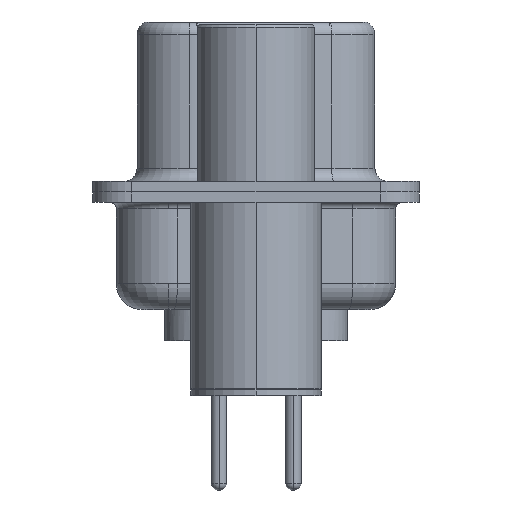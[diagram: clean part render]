
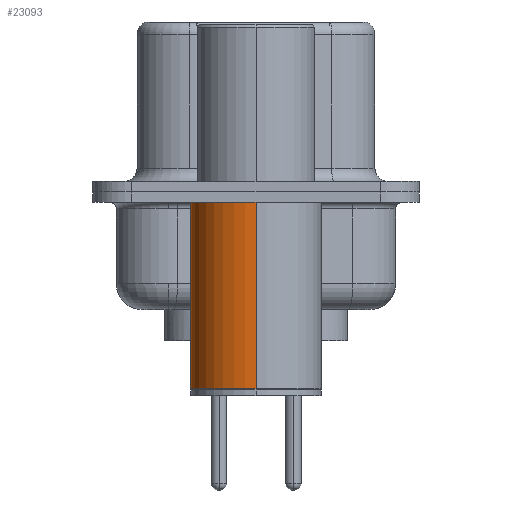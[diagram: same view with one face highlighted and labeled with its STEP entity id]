
A CAD part, left-side view. The second image highlights one B-rep face of the part: STEP entity #23093.
In plain terms, the highlighted cylindrical face has radius 2.5 mm (diameter 5 mm), a partial arc.
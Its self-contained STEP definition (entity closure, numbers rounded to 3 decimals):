
#487 = EDGE_CURVE ( 'NONE', #24582, #23290, #26613, .T. ) ;
#825 = CARTESIAN_POINT ( 'NONE',  ( 2.5, 0., -7.525 ) ) ;
#1726 = AXIS2_PLACEMENT_3D ( 'NONE', #17259, #23278, #4739 ) ;
#1856 = LINE ( 'NONE', #22162, #21550 ) ;
#3023 = CIRCLE ( 'NONE', #1726, 2.5 ) ;
#3059 = FACE_OUTER_BOUND ( 'NONE', #3855, .T. ) ;
#3647 = VERTEX_POINT ( 'NONE', #21560 ) ;
#3855 = EDGE_LOOP ( 'NONE', ( #4456, #26342, #9436, #11834 ) ) ;
#4138 = CARTESIAN_POINT ( 'NONE',  ( -2.5, 0., -0.4 ) ) ;
#4248 = VECTOR ( 'NONE', #20908, 1000. ) ;
#4456 = ORIENTED_EDGE ( 'NONE', *, *, #12412, .T. ) ;
#4544 = LINE ( 'NONE', #25258, #4248 ) ;
#4739 = DIRECTION ( 'NONE',  ( 1., 0., 0. ) ) ;
#4787 = EDGE_CURVE ( 'NONE', #20420, #24582, #4544, .T. ) ;
#4837 = CYLINDRICAL_SURFACE ( 'NONE', #8531, 2.5 ) ;
#8531 = AXIS2_PLACEMENT_3D ( 'NONE', #15748, #23914, #19706 ) ;
#9399 = CARTESIAN_POINT ( 'NONE',  ( 0., 0., -0.4 ) ) ;
#9436 = ORIENTED_EDGE ( 'NONE', *, *, #487, .F. ) ;
#11834 = ORIENTED_EDGE ( 'NONE', *, *, #4787, .F. ) ;
#12412 = EDGE_CURVE ( 'NONE', #20420, #3647, #3023, .T. ) ;
#13568 = AXIS2_PLACEMENT_3D ( 'NONE', #9399, #17707, #19908 ) ;
#15748 = CARTESIAN_POINT ( 'NONE',  ( 0., 0., 0.581 ) ) ;
#16295 = DIRECTION ( 'NONE',  ( 0., 0., 1. ) ) ;
#17259 = CARTESIAN_POINT ( 'NONE',  ( 0., 0., -7.525 ) ) ;
#17707 = DIRECTION ( 'NONE',  ( 0., 0., 1. ) ) ;
#18202 = CARTESIAN_POINT ( 'NONE',  ( 2.5, 0., -0.4 ) ) ;
#19706 = DIRECTION ( 'NONE',  ( 1., 0., 0. ) ) ;
#19908 = DIRECTION ( 'NONE',  ( 1., 0., 0. ) ) ;
#20420 = VERTEX_POINT ( 'NONE', #825 ) ;
#20908 = DIRECTION ( 'NONE',  ( 0., 0., 1. ) ) ;
#21303 = EDGE_CURVE ( 'NONE', #3647, #23290, #1856, .T. ) ;
#21550 = VECTOR ( 'NONE', #16295, 1000. ) ;
#21560 = CARTESIAN_POINT ( 'NONE',  ( -2.5, 0., -7.525 ) ) ;
#22162 = CARTESIAN_POINT ( 'NONE',  ( -2.5, 0., 0.581 ) ) ;
#23093 = ADVANCED_FACE ( 'NONE', ( #3059 ), #4837, .T. ) ;
#23278 = DIRECTION ( 'NONE',  ( 0., 0., 1. ) ) ;
#23290 = VERTEX_POINT ( 'NONE', #4138 ) ;
#23914 = DIRECTION ( 'NONE',  ( 0., 0., 1. ) ) ;
#24582 = VERTEX_POINT ( 'NONE', #18202 ) ;
#25258 = CARTESIAN_POINT ( 'NONE',  ( 2.5, 0., 0.581 ) ) ;
#26342 = ORIENTED_EDGE ( 'NONE', *, *, #21303, .T. ) ;
#26613 = CIRCLE ( 'NONE', #13568, 2.5 ) ;
